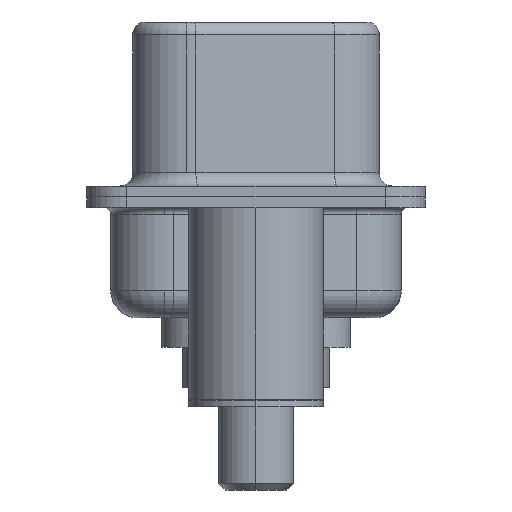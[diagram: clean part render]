
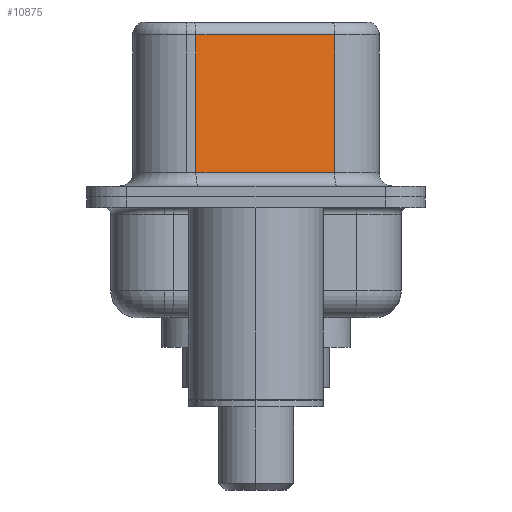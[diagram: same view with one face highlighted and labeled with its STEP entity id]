
A CAD part, left-side view. The second image highlights one B-rep face of the part: STEP entity #10875.
In plain terms, the highlighted planar face has unit normal (-0.985, -0.174, 0).
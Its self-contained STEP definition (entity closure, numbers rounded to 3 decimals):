
#61 = VECTOR ( 'NONE', #10337, 1000. ) ;
#339 = PLANE ( 'NONE',  #3776 ) ;
#943 = CARTESIAN_POINT ( 'NONE',  ( 4.585, -2.927, 0.9 ) ) ;
#1305 = DIRECTION ( 'NONE',  ( 0., 0., -1. ) ) ;
#1339 = EDGE_CURVE ( 'NONE', #12599, #8793, #5163, .T. ) ;
#1601 = DIRECTION ( 'NONE',  ( 0.985, 0.174, 0. ) ) ;
#1908 = VECTOR ( 'NONE', #1305, 1000. ) ;
#2555 = VERTEX_POINT ( 'NONE', #14422 ) ;
#3344 = LINE ( 'NONE', #3457, #61 ) ;
#3457 = CARTESIAN_POINT ( 'NONE',  ( 3.675, 2.233, 6.52 ) ) ;
#3776 = AXIS2_PLACEMENT_3D ( 'NONE', #8487, #1601, #9632 ) ;
#3912 = CARTESIAN_POINT ( 'NONE',  ( 3.675, 2.233, 0.9 ) ) ;
#4323 = VECTOR ( 'NONE', #8693, 1000. ) ;
#4787 = EDGE_CURVE ( 'NONE', #12599, #2555, #11050, .T. ) ;
#4805 = EDGE_CURVE ( 'NONE', #9992, #2555, #7297, .T. ) ;
#5163 = LINE ( 'NONE', #7216, #8089 ) ;
#5590 = DIRECTION ( 'NONE',  ( -0.174, 0.985, 0. ) ) ;
#7216 = CARTESIAN_POINT ( 'NONE',  ( 4.585, -2.927, 6.02 ) ) ;
#7297 = LINE ( 'NONE', #943, #4323 ) ;
#8089 = VECTOR ( 'NONE', #5590, 1000. ) ;
#8487 = CARTESIAN_POINT ( 'NONE',  ( 4.585, -2.927, 6.52 ) ) ;
#8693 = DIRECTION ( 'NONE',  ( 0.174, -0.985, 0. ) ) ;
#8726 = ORIENTED_EDGE ( 'NONE', *, *, #4787, .F. ) ;
#8793 = VERTEX_POINT ( 'NONE', #10350 ) ;
#9099 = EDGE_LOOP ( 'NONE', ( #8726, #11099, #14380, #13812 ) ) ;
#9632 = DIRECTION ( 'NONE',  ( -0.174, 0.985, 0. ) ) ;
#9760 = FACE_OUTER_BOUND ( 'NONE', #9099, .T. ) ;
#9992 = VERTEX_POINT ( 'NONE', #3912 ) ;
#10337 = DIRECTION ( 'NONE',  ( 0., 0., -1. ) ) ;
#10350 = CARTESIAN_POINT ( 'NONE',  ( 3.675, 2.233, 6.02 ) ) ;
#10875 = ADVANCED_FACE ( 'NONE', ( #9760 ), #339, .F. ) ;
#11050 = LINE ( 'NONE', #12932, #1908 ) ;
#11099 = ORIENTED_EDGE ( 'NONE', *, *, #1339, .T. ) ;
#11534 = CARTESIAN_POINT ( 'NONE',  ( 4.585, -2.927, 6.02 ) ) ;
#12599 = VERTEX_POINT ( 'NONE', #11534 ) ;
#12932 = CARTESIAN_POINT ( 'NONE',  ( 4.585, -2.927, 6.52 ) ) ;
#13372 = EDGE_CURVE ( 'NONE', #8793, #9992, #3344, .T. ) ;
#13812 = ORIENTED_EDGE ( 'NONE', *, *, #4805, .T. ) ;
#14380 = ORIENTED_EDGE ( 'NONE', *, *, #13372, .T. ) ;
#14422 = CARTESIAN_POINT ( 'NONE',  ( 4.585, -2.927, 0.9 ) ) ;
